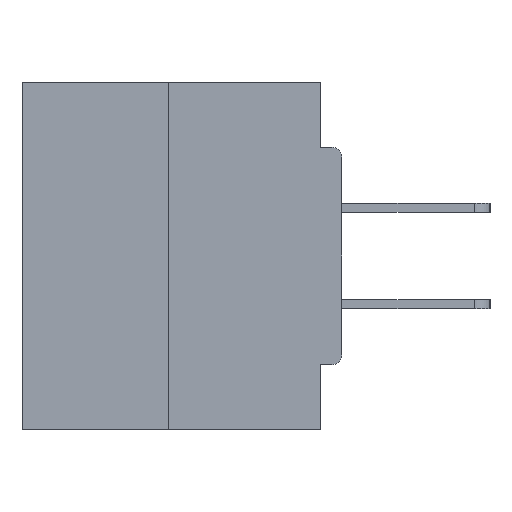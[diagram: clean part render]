
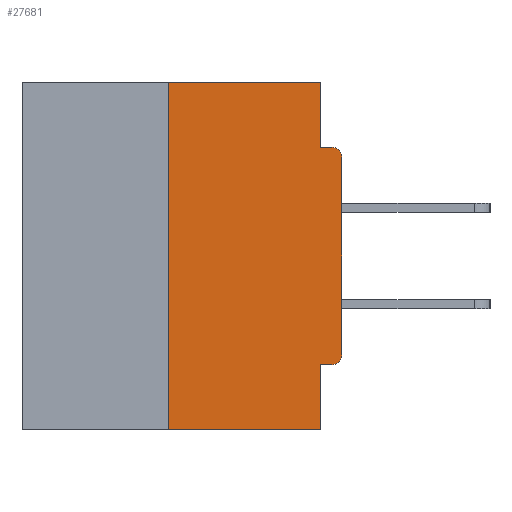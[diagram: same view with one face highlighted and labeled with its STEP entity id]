
A CAD part, left-side view. The second image highlights one B-rep face of the part: STEP entity #27681.
In plain terms, the highlighted planar face has unit normal (-1, 0, 0).
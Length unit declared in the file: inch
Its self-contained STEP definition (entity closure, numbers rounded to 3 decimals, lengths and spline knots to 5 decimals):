
#475 = CARTESIAN_POINT ( 'NONE',  ( 0., 0.46, -0.5 ) ) ;
#725 = DIRECTION ( 'NONE',  ( 0., 1., 0. ) ) ;
#917 = CARTESIAN_POINT ( 'NONE',  ( 0., 0., -0.3915 ) ) ;
#1340 = VECTOR ( 'NONE', #9953, 39.37008 ) ;
#2151 = CARTESIAN_POINT ( 'NONE',  ( 0., 0.031, -0.4065 ) ) ;
#3476 = CARTESIAN_POINT ( 'NONE',  ( 0., 0.015, -0.1085 ) ) ;
#3646 = DIRECTION ( 'NONE',  ( 0., 0., -1. ) ) ;
#3677 = CARTESIAN_POINT ( 'NONE',  ( 0., 0., -0.1085 ) ) ;
#4312 = EDGE_CURVE ( 'NONE', #31282, #24990, #11888, .T. ) ;
#4486 = EDGE_CURVE ( 'NONE', #18880, #28794, #8865, .T. ) ;
#4921 = DIRECTION ( 'NONE',  ( 0., -1., 0. ) ) ;
#5200 = VERTEX_POINT ( 'NONE', #34926 ) ;
#6362 = EDGE_CURVE ( 'NONE', #31313, #31282, #23051, .T. ) ;
#6603 = LINE ( 'NONE', #25854, #27407 ) ;
#6803 = VECTOR ( 'NONE', #24492, 39.37008 ) ;
#7002 = CARTESIAN_POINT ( 'NONE',  ( 0., 0., 0. ) ) ;
#8865 = LINE ( 'NONE', #25012, #24568 ) ;
#9953 = DIRECTION ( 'NONE',  ( 0., 0., 1. ) ) ;
#10169 = CARTESIAN_POINT ( 'NONE',  ( 0., 0., -0.0935 ) ) ;
#10246 = CARTESIAN_POINT ( 'NONE',  ( 0., 0.031, -0.0935 ) ) ;
#10306 = AXIS2_PLACEMENT_3D ( 'NONE', #34896, #32178, #10437 ) ;
#10437 = DIRECTION ( 'NONE',  ( 0., 0., -1. ) ) ;
#10959 = VERTEX_POINT ( 'NONE', #21393 ) ;
#11040 = CIRCLE ( 'NONE', #32533, 0.015 ) ;
#11293 = CARTESIAN_POINT ( 'NONE',  ( 0., 0.25, 0. ) ) ;
#11425 = DIRECTION ( 'NONE',  ( 0., 0., 1. ) ) ;
#11860 = EDGE_CURVE ( 'NONE', #10959, #25219, #19825, .T. ) ;
#11888 = CIRCLE ( 'NONE', #35009, 0.015 ) ;
#12443 = LINE ( 'NONE', #10169, #25563 ) ;
#13957 = DIRECTION ( 'NONE',  ( 0., -1., 0. ) ) ;
#15434 = ORIENTED_EDGE ( 'NONE', *, *, #35021, .F. ) ;
#18269 = CARTESIAN_POINT ( 'NONE',  ( 0., 0.015, -0.3915 ) ) ;
#18561 = EDGE_CURVE ( 'NONE', #25219, #31373, #24893, .T. ) ;
#18855 = ORIENTED_EDGE ( 'NONE', *, *, #6362, .T. ) ;
#18880 = VERTEX_POINT ( 'NONE', #2151 ) ;
#18975 = VECTOR ( 'NONE', #11425, 39.37008 ) ;
#19294 = DIRECTION ( 'NONE',  ( 0., 0., -1. ) ) ;
#19407 = CARTESIAN_POINT ( 'NONE',  ( 0., 0.25, 0. ) ) ;
#19825 = LINE ( 'NONE', #11293, #18975 ) ;
#20422 = LINE ( 'NONE', #475, #6803 ) ;
#20629 = ORIENTED_EDGE ( 'NONE', *, *, #18561, .F. ) ;
#20648 = DIRECTION ( 'NONE',  ( 0., 0., -1. ) ) ;
#20984 = DIRECTION ( 'NONE',  ( -1., 0., 0. ) ) ;
#21136 = VERTEX_POINT ( 'NONE', #10246 ) ;
#21266 = PLANE ( 'NONE',  #10306 ) ;
#21393 = CARTESIAN_POINT ( 'NONE',  ( 0., 0.25, -0.5 ) ) ;
#21762 = CARTESIAN_POINT ( 'NONE',  ( 0., 0.015, -0.0935 ) ) ;
#22439 = ORIENTED_EDGE ( 'NONE', *, *, #30594, .F. ) ;
#23051 = LINE ( 'NONE', #7002, #1340 ) ;
#23507 = ORIENTED_EDGE ( 'NONE', *, *, #29967, .F. ) ;
#24390 = EDGE_CURVE ( 'NONE', #5200, #31313, #11040, .T. ) ;
#24492 = DIRECTION ( 'NONE',  ( 0., -1., 0. ) ) ;
#24568 = VECTOR ( 'NONE', #3646, 39.37008 ) ;
#24618 = DIRECTION ( 'NONE',  ( -1., 0., 0. ) ) ;
#24786 = ORIENTED_EDGE ( 'NONE', *, *, #27238, .T. ) ;
#24893 = LINE ( 'NONE', #24975, #33840 ) ;
#24975 = CARTESIAN_POINT ( 'NONE',  ( 0., 0.46, 0. ) ) ;
#24990 = VERTEX_POINT ( 'NONE', #21762 ) ;
#25012 = CARTESIAN_POINT ( 'NONE',  ( 0., 0.031, -0.5 ) ) ;
#25087 = CARTESIAN_POINT ( 'NONE',  ( 0., 0., -0.4065 ) ) ;
#25219 = VERTEX_POINT ( 'NONE', #19407 ) ;
#25563 = VECTOR ( 'NONE', #4921, 39.37008 ) ;
#25839 = ORIENTED_EDGE ( 'NONE', *, *, #4486, .F. ) ;
#25854 = CARTESIAN_POINT ( 'NONE',  ( 0., 0.031, 0. ) ) ;
#26087 = LINE ( 'NONE', #25087, #26922 ) ;
#26266 = CARTESIAN_POINT ( 'NONE',  ( 0., 0.031, -0.5 ) ) ;
#26764 = DIRECTION ( 'NONE',  ( 0., 0., -1. ) ) ;
#26922 = VECTOR ( 'NONE', #725, 39.37008 ) ;
#27238 = EDGE_CURVE ( 'NONE', #10959, #28794, #20422, .T. ) ;
#27407 = VECTOR ( 'NONE', #20648, 39.37008 ) ;
#27681 = ADVANCED_FACE ( 'NONE', ( #29297 ), #21266, .F. ) ;
#27925 = ORIENTED_EDGE ( 'NONE', *, *, #4312, .T. ) ;
#28794 = VERTEX_POINT ( 'NONE', #26266 ) ;
#29297 = FACE_OUTER_BOUND ( 'NONE', #33059, .T. ) ;
#29967 = EDGE_CURVE ( 'NONE', #31373, #21136, #6603, .T. ) ;
#30594 = EDGE_CURVE ( 'NONE', #5200, #18880, #26087, .T. ) ;
#31282 = VERTEX_POINT ( 'NONE', #3677 ) ;
#31313 = VERTEX_POINT ( 'NONE', #917 ) ;
#31345 = CARTESIAN_POINT ( 'NONE',  ( 0., 0.031, 0. ) ) ;
#31373 = VERTEX_POINT ( 'NONE', #31345 ) ;
#31711 = ORIENTED_EDGE ( 'NONE', *, *, #24390, .T. ) ;
#32178 = DIRECTION ( 'NONE',  ( 1., 0., 0. ) ) ;
#32187 = ORIENTED_EDGE ( 'NONE', *, *, #11860, .F. ) ;
#32533 = AXIS2_PLACEMENT_3D ( 'NONE', #18269, #20984, #26764 ) ;
#33059 = EDGE_LOOP ( 'NONE', ( #20629, #32187, #24786, #25839, #22439, #31711, #18855, #27925, #15434, #23507 ) ) ;
#33840 = VECTOR ( 'NONE', #13957, 39.37008 ) ;
#34896 = CARTESIAN_POINT ( 'NONE',  ( 0., 0.46, 0. ) ) ;
#34926 = CARTESIAN_POINT ( 'NONE',  ( 0., 0.015, -0.4065 ) ) ;
#35009 = AXIS2_PLACEMENT_3D ( 'NONE', #3476, #24618, #19294 ) ;
#35021 = EDGE_CURVE ( 'NONE', #21136, #24990, #12443, .T. ) ;
